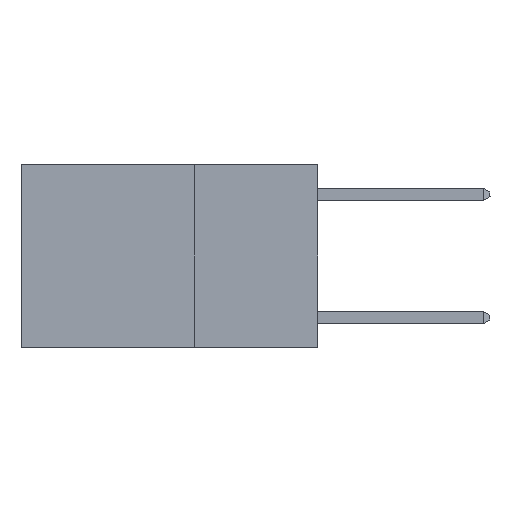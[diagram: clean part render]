
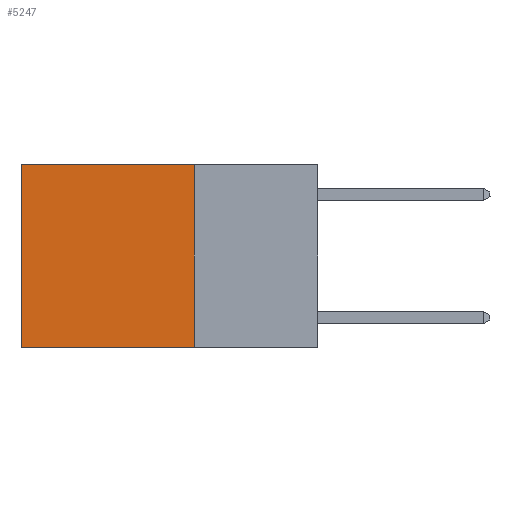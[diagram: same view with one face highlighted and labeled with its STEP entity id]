
A CAD part, left-side view. The second image highlights one B-rep face of the part: STEP entity #5247.
In plain terms, the highlighted planar face has unit normal (-1, 0, 0).
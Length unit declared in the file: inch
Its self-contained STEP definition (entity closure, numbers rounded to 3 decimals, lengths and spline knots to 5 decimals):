
#527 = ORIENTED_EDGE ( 'NONE', *, *, #3872, .T. ) ;
#1294 = CARTESIAN_POINT ( 'NONE',  ( 0.2625, 0.6, 0. ) ) ;
#1532 = FACE_OUTER_BOUND ( 'NONE', #11411, .T. ) ;
#2085 = DIRECTION ( 'NONE',  ( 1., 0., 0. ) ) ;
#3115 = VECTOR ( 'NONE', #14995, 39.37008 ) ;
#3128 = CARTESIAN_POINT ( 'NONE',  ( 0.2625, 0.25, 0. ) ) ;
#3872 = EDGE_CURVE ( 'NONE', #12348, #8969, #14967, .T. ) ;
#4017 = EDGE_CURVE ( 'NONE', #6520, #12348, #11523, .T. ) ;
#4737 = CARTESIAN_POINT ( 'NONE',  ( 0.2625, 0.25, -0.37 ) ) ;
#5041 = EDGE_CURVE ( 'NONE', #8794, #8969, #10709, .T. ) ;
#5228 = CARTESIAN_POINT ( 'NONE',  ( 0.2625, 0.6, -0.37 ) ) ;
#5247 = ADVANCED_FACE ( 'NONE', ( #1532 ), #14739, .F. ) ;
#5727 = CARTESIAN_POINT ( 'NONE',  ( 0.2625, 0.25, 0. ) ) ;
#6243 = CARTESIAN_POINT ( 'NONE',  ( 0.2625, 0.25, 0. ) ) ;
#6374 = CARTESIAN_POINT ( 'NONE',  ( 0.2625, 0.25, -0.37 ) ) ;
#6446 = CARTESIAN_POINT ( 'NONE',  ( 0.2625, 0.25, 0. ) ) ;
#6520 = VERTEX_POINT ( 'NONE', #3128 ) ;
#6575 = ORIENTED_EDGE ( 'NONE', *, *, #5041, .F. ) ;
#6887 = LINE ( 'NONE', #6243, #12521 ) ;
#7196 = CARTESIAN_POINT ( 'NONE',  ( 0.2625, 0.6, 0. ) ) ;
#7366 = ORIENTED_EDGE ( 'NONE', *, *, #4017, .T. ) ;
#7393 = DIRECTION ( 'NONE',  ( 0., 0., -1. ) ) ;
#8794 = VERTEX_POINT ( 'NONE', #4737 ) ;
#8969 = VERTEX_POINT ( 'NONE', #5228 ) ;
#9738 = AXIS2_PLACEMENT_3D ( 'NONE', #5727, #2085, #10338 ) ;
#9834 = ORIENTED_EDGE ( 'NONE', *, *, #11538, .F. ) ;
#10338 = DIRECTION ( 'NONE',  ( 0., 0., -1. ) ) ;
#10709 = LINE ( 'NONE', #6374, #14015 ) ;
#11164 = VECTOR ( 'NONE', #13179, 39.37008 ) ;
#11411 = EDGE_LOOP ( 'NONE', ( #527, #6575, #9834, #7366 ) ) ;
#11523 = LINE ( 'NONE', #6446, #11164 ) ;
#11538 = EDGE_CURVE ( 'NONE', #6520, #8794, #6887, .T. ) ;
#12348 = VERTEX_POINT ( 'NONE', #1294 ) ;
#12521 = VECTOR ( 'NONE', #7393, 39.37008 ) ;
#13179 = DIRECTION ( 'NONE',  ( 0., 1., 0. ) ) ;
#14015 = VECTOR ( 'NONE', #14236, 39.37008 ) ;
#14236 = DIRECTION ( 'NONE',  ( 0., 1., 0. ) ) ;
#14739 = PLANE ( 'NONE',  #9738 ) ;
#14967 = LINE ( 'NONE', #7196, #3115 ) ;
#14995 = DIRECTION ( 'NONE',  ( 0., 0., -1. ) ) ;
